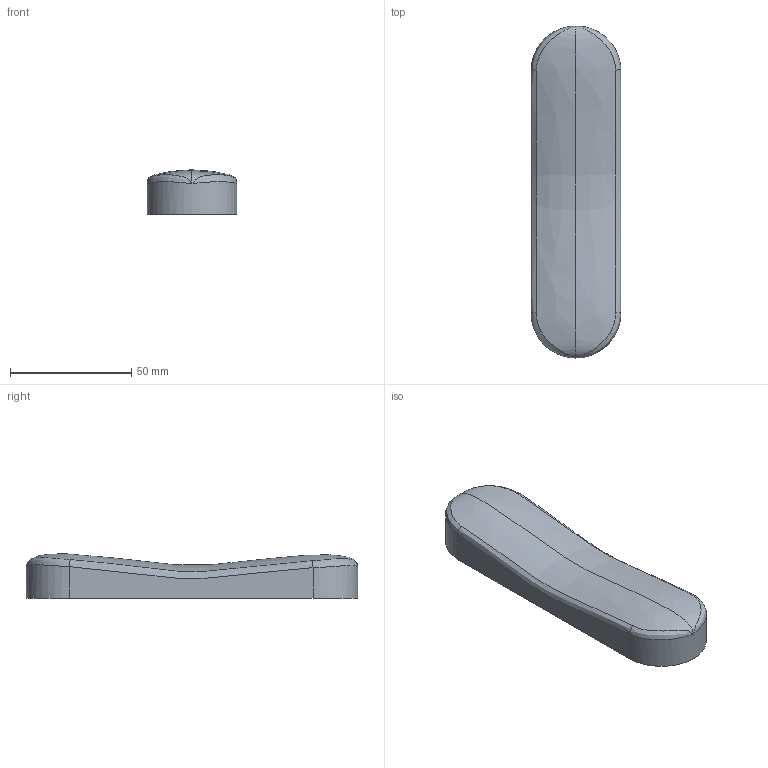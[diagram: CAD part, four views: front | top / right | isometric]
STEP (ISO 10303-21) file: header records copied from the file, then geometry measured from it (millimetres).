
FILE_DESCRIPTION (( 'STEP AP214' ), '1' );
FILE_NAME ('Rifle_Butt_Pad.STEP', '2013-09-01T16:43:10', ( 'Asher' ), ( '' ), 'SwSTEP 2.0', 'SolidWorks 2013', '' );
FILE_SCHEMA (( 'AUTOMOTIVE_DESIGN' ));
Length unit declared in the file: millimetre
Products named in the file (1): Rifle_Butt_Pad
Bounding box: 37.13 x 137.04 x 18.3 mm (x, y, z)
Volume: 71264.8 mm3; surface area: 14066.2 mm2
Topology: 1 solids, 1 shells, 19 faces, 45 edges, 26 vertices
Faces by surface type: bspline 8, cylinder 6, plane 5
Entity records: 2672 total; most frequent: CARTESIAN_POINT 2280, ORIENTED_EDGE 82, DIRECTION 58, EDGE_CURVE 41, VERTEX_POINT 26, AXIS2_PLACEMENT_3D 24, EDGE_LOOP 21, ADVANCED_FACE 19
